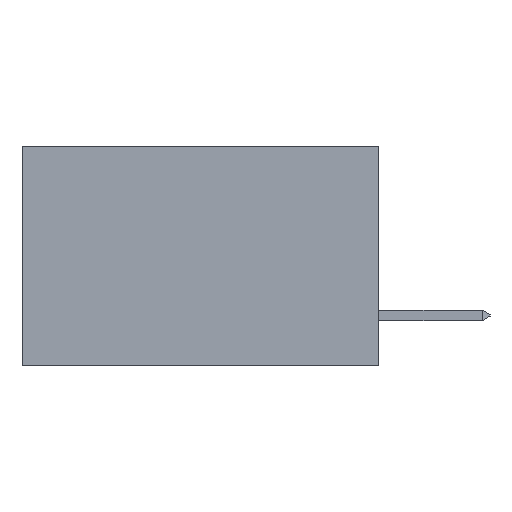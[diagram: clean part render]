
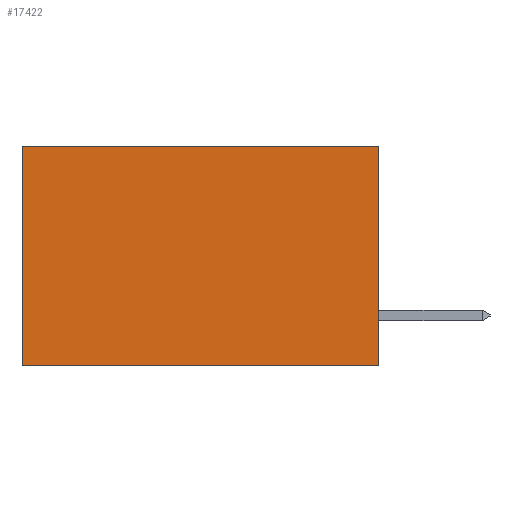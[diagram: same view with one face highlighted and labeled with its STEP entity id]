
A CAD part, left-side view. The second image highlights one B-rep face of the part: STEP entity #17422.
In plain terms, the highlighted planar face has unit normal (-1, 0, 0).
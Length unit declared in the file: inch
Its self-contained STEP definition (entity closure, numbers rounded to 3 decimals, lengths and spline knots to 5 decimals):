
#858 = EDGE_CURVE ( 'NONE', #5808, #20214, #2419, .T. ) ;
#1229 = DIRECTION ( 'NONE',  ( 1., 0., 0. ) ) ;
#2419 = LINE ( 'NONE', #3285, #10850 ) ;
#3228 = DIRECTION ( 'NONE',  ( 0., 1., 0. ) ) ;
#3285 = CARTESIAN_POINT ( 'NONE',  ( 0.298, 0., 0. ) ) ;
#3633 = CARTESIAN_POINT ( 'NONE',  ( 0.298, 0.6, -0.37 ) ) ;
#3856 = DIRECTION ( 'NONE',  ( 0., 0., -1. ) ) ;
#5244 = ORIENTED_EDGE ( 'NONE', *, *, #8802, .T. ) ;
#5808 = VERTEX_POINT ( 'NONE', #8628 ) ;
#6210 = FACE_OUTER_BOUND ( 'NONE', #10591, .T. ) ;
#6693 = VECTOR ( 'NONE', #3228, 39.37008 ) ;
#6984 = VECTOR ( 'NONE', #3856, 39.37008 ) ;
#7439 = ORIENTED_EDGE ( 'NONE', *, *, #18234, .F. ) ;
#7529 = CARTESIAN_POINT ( 'NONE',  ( 0.298, 0., 0. ) ) ;
#7871 = CARTESIAN_POINT ( 'NONE',  ( 0.298, 0., 0. ) ) ;
#8628 = CARTESIAN_POINT ( 'NONE',  ( 0.298, 0., 0. ) ) ;
#8802 = EDGE_CURVE ( 'NONE', #12340, #18948, #11526, .T. ) ;
#9335 = DIRECTION ( 'NONE',  ( 0., 1., 0. ) ) ;
#9582 = PLANE ( 'NONE',  #10806 ) ;
#9755 = CARTESIAN_POINT ( 'NONE',  ( 0.298, 0.6, 0. ) ) ;
#10591 = EDGE_LOOP ( 'NONE', ( #5244, #7439, #17913, #14995 ) ) ;
#10630 = LINE ( 'NONE', #7529, #19106 ) ;
#10806 = AXIS2_PLACEMENT_3D ( 'NONE', #7871, #1229, #13027 ) ;
#10850 = VECTOR ( 'NONE', #14201, 39.37008 ) ;
#11241 = EDGE_CURVE ( 'NONE', #5808, #12340, #10630, .T. ) ;
#11526 = LINE ( 'NONE', #14032, #6984 ) ;
#12340 = VERTEX_POINT ( 'NONE', #9755 ) ;
#13027 = DIRECTION ( 'NONE',  ( 0., 0., -1. ) ) ;
#14032 = CARTESIAN_POINT ( 'NONE',  ( 0.298, 0.6, 0. ) ) ;
#14201 = DIRECTION ( 'NONE',  ( 0., 0., -1. ) ) ;
#14995 = ORIENTED_EDGE ( 'NONE', *, *, #11241, .T. ) ;
#16718 = CARTESIAN_POINT ( 'NONE',  ( 0.298, 0., -0.37 ) ) ;
#17422 = ADVANCED_FACE ( 'NONE', ( #6210 ), #9582, .F. ) ;
#17913 = ORIENTED_EDGE ( 'NONE', *, *, #858, .F. ) ;
#18234 = EDGE_CURVE ( 'NONE', #20214, #18948, #20229, .T. ) ;
#18457 = CARTESIAN_POINT ( 'NONE',  ( 0.298, 0., -0.37 ) ) ;
#18948 = VERTEX_POINT ( 'NONE', #3633 ) ;
#19106 = VECTOR ( 'NONE', #9335, 39.37008 ) ;
#20214 = VERTEX_POINT ( 'NONE', #16718 ) ;
#20229 = LINE ( 'NONE', #18457, #6693 ) ;
